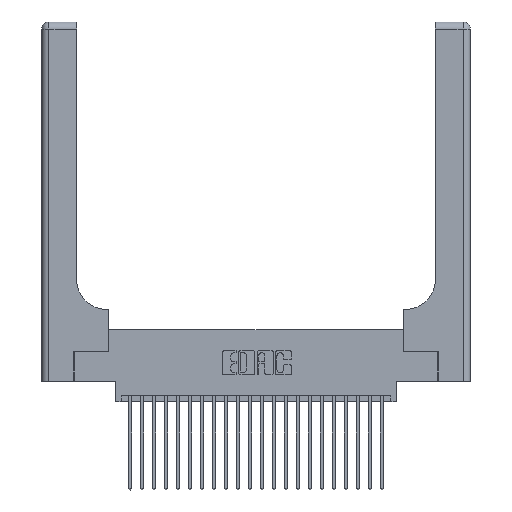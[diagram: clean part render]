
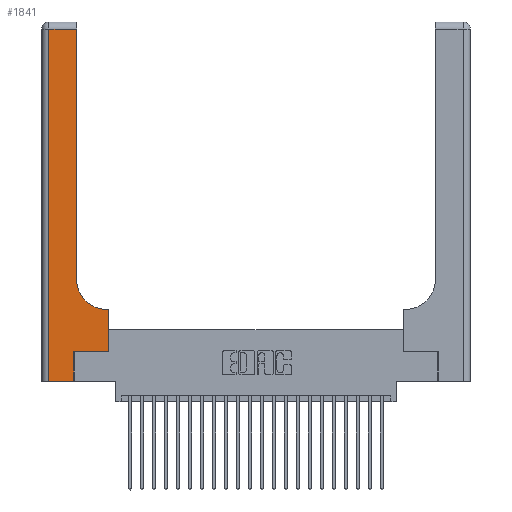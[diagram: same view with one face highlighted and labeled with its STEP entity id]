
A CAD part, top view. The second image highlights one B-rep face of the part: STEP entity #1841.
In plain terms, the highlighted planar face has unit normal (0, 0, 1).
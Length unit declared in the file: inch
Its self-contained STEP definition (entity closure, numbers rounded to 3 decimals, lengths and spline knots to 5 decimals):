
#126 = VECTOR ( 'NONE', #5423, 39.37008 ) ;
#350 = CARTESIAN_POINT ( 'NONE',  ( 0.5585, 0.6, 0.37 ) ) ;
#1242 = CARTESIAN_POINT ( 'NONE',  ( 0.2915, 0.85, 0.37 ) ) ;
#1476 = CARTESIAN_POINT ( 'NONE',  ( 0.269, 0.25, 0.37 ) ) ;
#1776 = LINE ( 'NONE', #7898, #5143 ) ;
#1841 = ADVANCED_FACE ( 'NONE', ( #5093 ), #24642, .F. ) ;
#1964 = LINE ( 'NONE', #5488, #126 ) ;
#2788 = EDGE_CURVE ( 'NONE', #14819, #17539, #5383, .T. ) ;
#3852 = EDGE_CURVE ( 'NONE', #22466, #17413, #1964, .T. ) ;
#3878 = CARTESIAN_POINT ( 'NONE',  ( 0.06, 2.94, 0.37 ) ) ;
#4175 = EDGE_CURVE ( 'NONE', #19535, #22466, #9558, .T. ) ;
#5077 = ORIENTED_EDGE ( 'NONE', *, *, #2788, .T. ) ;
#5093 = FACE_OUTER_BOUND ( 'NONE', #15440, .T. ) ;
#5143 = VECTOR ( 'NONE', #17657, 39.37008 ) ;
#5236 = CARTESIAN_POINT ( 'NONE',  ( 0., 3., 0.37 ) ) ;
#5383 = LINE ( 'NONE', #7137, #21899 ) ;
#5423 = DIRECTION ( 'NONE',  ( 0., 1., 0. ) ) ;
#5488 = CARTESIAN_POINT ( 'NONE',  ( 0.2915, 3., 0.37 ) ) ;
#5876 = CARTESIAN_POINT ( 'NONE',  ( 0.269, 0., 0.37 ) ) ;
#6951 = EDGE_CURVE ( 'NONE', #17413, #22942, #7983, .T. ) ;
#7137 = CARTESIAN_POINT ( 'NONE',  ( 0.269, 0., 0.37 ) ) ;
#7510 = VERTEX_POINT ( 'NONE', #14849 ) ;
#7652 = LINE ( 'NONE', #10995, #22634 ) ;
#7683 = ORIENTED_EDGE ( 'NONE', *, *, #4175, .T. ) ;
#7898 = CARTESIAN_POINT ( 'NONE',  ( 0.5585, 0.25, 0.37 ) ) ;
#7983 = LINE ( 'NONE', #23567, #25133 ) ;
#8072 = CARTESIAN_POINT ( 'NONE',  ( 0.06, 3., 0.37 ) ) ;
#8567 = EDGE_CURVE ( 'NONE', #25105, #19535, #7652, .T. ) ;
#8730 = AXIS2_PLACEMENT_3D ( 'NONE', #5236, #16846, #16687 ) ;
#9558 = CIRCLE ( 'NONE', #17694, 0.25 ) ;
#9731 = EDGE_CURVE ( 'NONE', #17539, #16325, #24102, .T. ) ;
#10045 = DIRECTION ( 'NONE',  ( -1., 0., 0. ) ) ;
#10995 = CARTESIAN_POINT ( 'NONE',  ( 0.2915, 0.6, 0.37 ) ) ;
#11393 = ORIENTED_EDGE ( 'NONE', *, *, #8567, .T. ) ;
#11487 = DIRECTION ( 'NONE',  ( 1., 0., 0. ) ) ;
#12052 = EDGE_CURVE ( 'NONE', #7510, #14819, #14912, .T. ) ;
#13103 = EDGE_CURVE ( 'NONE', #22942, #7510, #16696, .T. ) ;
#13781 = CARTESIAN_POINT ( 'NONE',  ( 0.5415, 0.6, 0.37 ) ) ;
#14474 = ORIENTED_EDGE ( 'NONE', *, *, #18356, .T. ) ;
#14819 = VERTEX_POINT ( 'NONE', #5876 ) ;
#14849 = CARTESIAN_POINT ( 'NONE',  ( 0.06, 0., 0.37 ) ) ;
#14912 = LINE ( 'NONE', #18289, #17670 ) ;
#15440 = EDGE_LOOP ( 'NONE', ( #18748, #15863, #18125, #19363, #5077, #19078, #14474, #11393, #7683 ) ) ;
#15863 = ORIENTED_EDGE ( 'NONE', *, *, #6951, .T. ) ;
#16151 = DIRECTION ( 'NONE',  ( 1., 0., 0. ) ) ;
#16325 = VERTEX_POINT ( 'NONE', #18900 ) ;
#16687 = DIRECTION ( 'NONE',  ( -1., 0., 0. ) ) ;
#16696 = LINE ( 'NONE', #8072, #24651 ) ;
#16846 = DIRECTION ( 'NONE',  ( 0., 0., -1. ) ) ;
#17092 = DIRECTION ( 'NONE',  ( -1., 0., 0. ) ) ;
#17225 = CARTESIAN_POINT ( 'NONE',  ( 0.5415, 0.85, 0.37 ) ) ;
#17413 = VERTEX_POINT ( 'NONE', #18431 ) ;
#17539 = VERTEX_POINT ( 'NONE', #24691 ) ;
#17657 = DIRECTION ( 'NONE',  ( 0., 1., 0. ) ) ;
#17665 = DIRECTION ( 'NONE',  ( 0., 0., -1. ) ) ;
#17670 = VECTOR ( 'NONE', #16151, 39.37008 ) ;
#17694 = AXIS2_PLACEMENT_3D ( 'NONE', #17225, #17665, #11487 ) ;
#18125 = ORIENTED_EDGE ( 'NONE', *, *, #13103, .T. ) ;
#18289 = CARTESIAN_POINT ( 'NONE',  ( 0., 0., 0.37 ) ) ;
#18356 = EDGE_CURVE ( 'NONE', #16325, #25105, #1776, .T. ) ;
#18431 = CARTESIAN_POINT ( 'NONE',  ( 0.2915, 2.94, 0.37 ) ) ;
#18748 = ORIENTED_EDGE ( 'NONE', *, *, #3852, .T. ) ;
#18900 = CARTESIAN_POINT ( 'NONE',  ( 0.5585, 0.25, 0.37 ) ) ;
#19078 = ORIENTED_EDGE ( 'NONE', *, *, #9731, .T. ) ;
#19363 = ORIENTED_EDGE ( 'NONE', *, *, #12052, .T. ) ;
#19535 = VERTEX_POINT ( 'NONE', #13781 ) ;
#21899 = VECTOR ( 'NONE', #22264, 39.37008 ) ;
#22264 = DIRECTION ( 'NONE',  ( 0., 1., 0. ) ) ;
#22268 = VECTOR ( 'NONE', #22732, 39.37008 ) ;
#22466 = VERTEX_POINT ( 'NONE', #1242 ) ;
#22634 = VECTOR ( 'NONE', #17092, 39.37008 ) ;
#22732 = DIRECTION ( 'NONE',  ( 1., 0., 0. ) ) ;
#22942 = VERTEX_POINT ( 'NONE', #3878 ) ;
#23567 = CARTESIAN_POINT ( 'NONE',  ( 0., 2.94, 0.37 ) ) ;
#23865 = DIRECTION ( 'NONE',  ( 0., -1., 0. ) ) ;
#24102 = LINE ( 'NONE', #1476, #22268 ) ;
#24642 = PLANE ( 'NONE',  #8730 ) ;
#24651 = VECTOR ( 'NONE', #23865, 39.37008 ) ;
#24691 = CARTESIAN_POINT ( 'NONE',  ( 0.269, 0.25, 0.37 ) ) ;
#25105 = VERTEX_POINT ( 'NONE', #350 ) ;
#25133 = VECTOR ( 'NONE', #10045, 39.37008 ) ;
